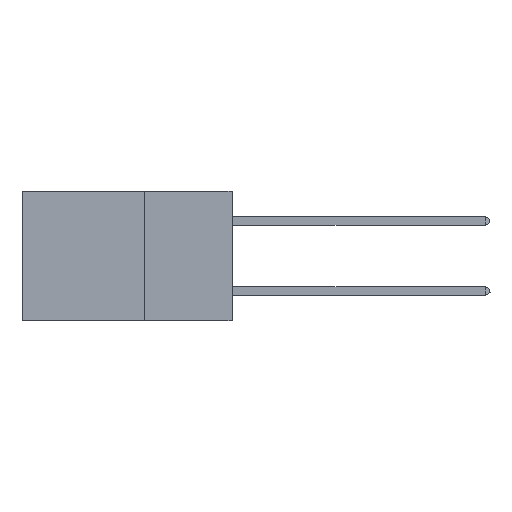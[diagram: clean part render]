
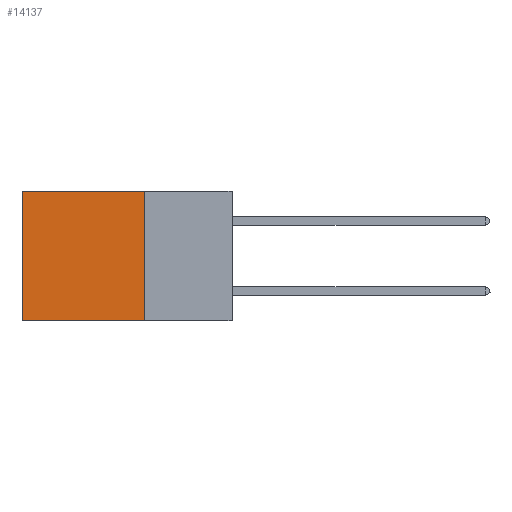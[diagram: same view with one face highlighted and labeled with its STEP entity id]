
A CAD part, left-side view. The second image highlights one B-rep face of the part: STEP entity #14137.
In plain terms, the highlighted planar face has unit normal (-1, 0, 0).
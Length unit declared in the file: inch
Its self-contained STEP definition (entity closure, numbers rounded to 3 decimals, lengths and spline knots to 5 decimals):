
#38 = CARTESIAN_POINT ( 'NONE',  ( 0.2875, 0.25, 0. ) ) ;
#308 = CARTESIAN_POINT ( 'NONE',  ( 0.2875, 0.25, -0.37 ) ) ;
#344 = CARTESIAN_POINT ( 'NONE',  ( 0.2875, 0.25, 0. ) ) ;
#408 = EDGE_LOOP ( 'NONE', ( #6966, #6467, #8169, #5072 ) ) ;
#793 = EDGE_CURVE ( 'NONE', #11984, #7550, #874, .T. ) ;
#848 = CARTESIAN_POINT ( 'NONE',  ( 0.2875, 0.6, 0. ) ) ;
#874 = LINE ( 'NONE', #1513, #13343 ) ;
#1060 = FACE_OUTER_BOUND ( 'NONE', #408, .T. ) ;
#1120 = VERTEX_POINT ( 'NONE', #38 ) ;
#1513 = CARTESIAN_POINT ( 'NONE',  ( 0.2875, 0.25, -0.37 ) ) ;
#1583 = DIRECTION ( 'NONE',  ( 1., 0., 0. ) ) ;
#2041 = CARTESIAN_POINT ( 'NONE',  ( 0.2875, 0.25, 0. ) ) ;
#2301 = EDGE_CURVE ( 'NONE', #1120, #11984, #5841, .T. ) ;
#2942 = DIRECTION ( 'NONE',  ( 0., 1., 0. ) ) ;
#3446 = EDGE_CURVE ( 'NONE', #1120, #5822, #9082, .T. ) ;
#3930 = VECTOR ( 'NONE', #4568, 39.37008 ) ;
#4080 = PLANE ( 'NONE',  #15781 ) ;
#4568 = DIRECTION ( 'NONE',  ( 0., 0., -1. ) ) ;
#5022 = CARTESIAN_POINT ( 'NONE',  ( 0.2875, 0.6, -0.37 ) ) ;
#5072 = ORIENTED_EDGE ( 'NONE', *, *, #3446, .T. ) ;
#5763 = DIRECTION ( 'NONE',  ( 0., 0., -1. ) ) ;
#5822 = VERTEX_POINT ( 'NONE', #5934 ) ;
#5841 = LINE ( 'NONE', #2041, #13904 ) ;
#5934 = CARTESIAN_POINT ( 'NONE',  ( 0.2875, 0.6, 0. ) ) ;
#6467 = ORIENTED_EDGE ( 'NONE', *, *, #793, .F. ) ;
#6579 = VECTOR ( 'NONE', #2942, 39.37008 ) ;
#6966 = ORIENTED_EDGE ( 'NONE', *, *, #7845, .T. ) ;
#7006 = LINE ( 'NONE', #848, #3930 ) ;
#7550 = VERTEX_POINT ( 'NONE', #5022 ) ;
#7845 = EDGE_CURVE ( 'NONE', #5822, #7550, #7006, .T. ) ;
#8169 = ORIENTED_EDGE ( 'NONE', *, *, #2301, .F. ) ;
#9082 = LINE ( 'NONE', #13942, #6579 ) ;
#10111 = DIRECTION ( 'NONE',  ( 0., 1., 0. ) ) ;
#10281 = DIRECTION ( 'NONE',  ( 0., 0., -1. ) ) ;
#11984 = VERTEX_POINT ( 'NONE', #308 ) ;
#13343 = VECTOR ( 'NONE', #10111, 39.37008 ) ;
#13904 = VECTOR ( 'NONE', #5763, 39.37008 ) ;
#13942 = CARTESIAN_POINT ( 'NONE',  ( 0.2875, 0.25, 0. ) ) ;
#14137 = ADVANCED_FACE ( 'NONE', ( #1060 ), #4080, .F. ) ;
#15781 = AXIS2_PLACEMENT_3D ( 'NONE', #344, #1583, #10281 ) ;
